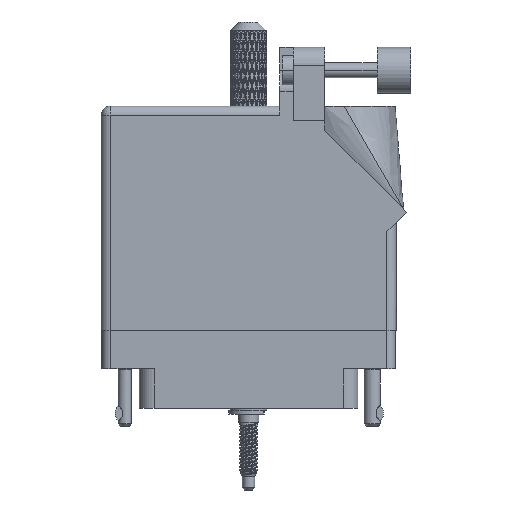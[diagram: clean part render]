
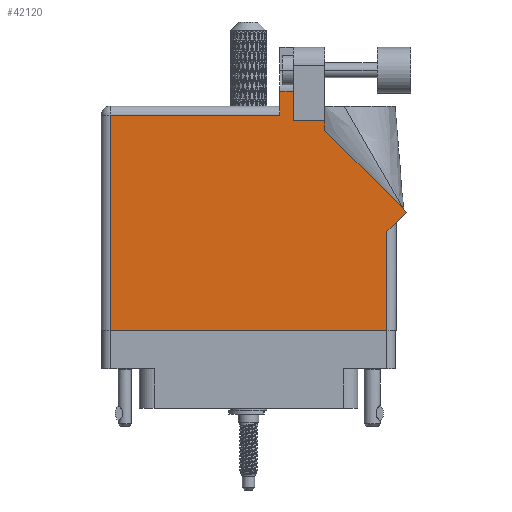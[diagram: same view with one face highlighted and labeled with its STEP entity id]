
A CAD part, front view. The second image highlights one B-rep face of the part: STEP entity #42120.
In plain terms, the highlighted face is planar.
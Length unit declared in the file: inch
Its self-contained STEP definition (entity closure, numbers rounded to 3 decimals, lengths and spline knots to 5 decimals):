
#35 = LINE ( 'NONE', #107461, #18611 ) ;
#295 = VECTOR ( 'NONE', #54217, 39.37008 ) ;
#3095 = ORIENTED_EDGE ( 'NONE', *, *, #90571, .T. ) ;
#4260 = VECTOR ( 'NONE', #101979, 39.37008 ) ;
#4283 = EDGE_CURVE ( 'NONE', #41379, #85957, #13879, .T. ) ;
#4672 = EDGE_LOOP ( 'NONE', ( #17886, #47079, #49174, #107931, #3095, #56860, #93008, #79670, #86311, #7730, #45377 ) ) ;
#5504 = EDGE_CURVE ( 'NONE', #63545, #100131, #31183, .T. ) ;
#6897 = EDGE_CURVE ( 'NONE', #9833, #75771, #57679, .T. ) ;
#7074 = DIRECTION ( 'NONE',  ( -0.707, 0.707, 0. ) ) ;
#7730 = ORIENTED_EDGE ( 'NONE', *, *, #89425, .T. ) ;
#8546 = CARTESIAN_POINT ( 'NONE',  ( 1.311, 1.6315, 0. ) ) ;
#9789 = CARTESIAN_POINT ( 'NONE',  ( 1.311, 1.43, 0. ) ) ;
#9833 = VERTEX_POINT ( 'NONE', #64422 ) ;
#13066 = CARTESIAN_POINT ( 'NONE',  ( 2.08071, 0.80771, 0. ) ) ;
#13879 = LINE ( 'NONE', #101035, #41938 ) ;
#14260 = FACE_OUTER_BOUND ( 'NONE', #4672, .T. ) ;
#17886 = ORIENTED_EDGE ( 'NONE', *, *, #5504, .T. ) ;
#18052 = DIRECTION ( 'NONE',  ( 0., 1., 0. ) ) ;
#18611 = VECTOR ( 'NONE', #90372, 39.37008 ) ;
#20107 = DIRECTION ( 'NONE',  ( 0., 0., -1. ) ) ;
#24949 = DIRECTION ( 'NONE',  ( -1., 0., 0. ) ) ;
#25776 = VECTOR ( 'NONE', #74172, 39.37008 ) ;
#29349 = CARTESIAN_POINT ( 'NONE',  ( 1.948, 0., 0. ) ) ;
#31183 = LINE ( 'NONE', #9789, #91169 ) ;
#32464 = VECTOR ( 'NONE', #33419, 39.37008 ) ;
#33419 = DIRECTION ( 'NONE',  ( -1., 0., 0. ) ) ;
#33654 = EDGE_CURVE ( 'NONE', #85957, #91461, #76544, .T. ) ;
#33769 = CARTESIAN_POINT ( 'NONE',  ( 0., 1.468, 0. ) ) ;
#35671 = EDGE_CURVE ( 'NONE', #63748, #59970, #40245, .T. ) ;
#40245 = LINE ( 'NONE', #63122, #295 ) ;
#41379 = VERTEX_POINT ( 'NONE', #47139 ) ;
#41938 = VECTOR ( 'NONE', #84261, 39.37008 ) ;
#42120 = ADVANCED_FACE ( 'NONE', ( #14260 ), #53612, .F. ) ;
#44382 = CARTESIAN_POINT ( 'NONE',  ( 1.217, 1.468, 0. ) ) ;
#45377 = ORIENTED_EDGE ( 'NONE', *, *, #84362, .T. ) ;
#45420 = CARTESIAN_POINT ( 'NONE',  ( 1.311, 1.43, 0. ) ) ;
#47079 = ORIENTED_EDGE ( 'NONE', *, *, #77019, .T. ) ;
#47139 = CARTESIAN_POINT ( 'NONE',  ( 1.217, 1.6315, 0. ) ) ;
#48373 = DIRECTION ( 'NONE',  ( -1., 0., 0. ) ) ;
#48534 = CARTESIAN_POINT ( 'NONE',  ( 0., 0., 0. ) ) ;
#49151 = CARTESIAN_POINT ( 'NONE',  ( 1.524, 1.36442, 0. ) ) ;
#49174 = ORIENTED_EDGE ( 'NONE', *, *, #4283, .T. ) ;
#53612 = PLANE ( 'NONE',  #97197 ) ;
#54217 = DIRECTION ( 'NONE',  ( 0.707, 0.707, 0. ) ) ;
#56860 = ORIENTED_EDGE ( 'NONE', *, *, #6897, .T. ) ;
#57381 = CARTESIAN_POINT ( 'NONE',  ( 2.08071, 0.80771, 0. ) ) ;
#57679 = LINE ( 'NONE', #48534, #98996 ) ;
#59598 = EDGE_CURVE ( 'NONE', #75771, #63748, #35, .T. ) ;
#59970 = VERTEX_POINT ( 'NONE', #13066 ) ;
#61467 = DIRECTION ( 'NONE',  ( -1., 0., 0. ) ) ;
#63122 = CARTESIAN_POINT ( 'NONE',  ( 2.01, 0.737, 0. ) ) ;
#63545 = VERTEX_POINT ( 'NONE', #45420 ) ;
#63748 = VERTEX_POINT ( 'NONE', #93444 ) ;
#64422 = CARTESIAN_POINT ( 'NONE',  ( 0.062, 0., 0. ) ) ;
#66461 = LINE ( 'NONE', #57381, #101136 ) ;
#68892 = CARTESIAN_POINT ( 'NONE',  ( 1.524, 1.43, 0. ) ) ;
#69588 = LINE ( 'NONE', #110540, #4260 ) ;
#71134 = CARTESIAN_POINT ( 'NONE',  ( 0., 1.53, 0. ) ) ;
#72449 = LINE ( 'NONE', #74529, #97967 ) ;
#72741 = VECTOR ( 'NONE', #24949, 39.37008 ) ;
#74172 = DIRECTION ( 'NONE',  ( 0., 1., 0. ) ) ;
#74529 = CARTESIAN_POINT ( 'NONE',  ( 1.64177, 1.6315, 0. ) ) ;
#75771 = VERTEX_POINT ( 'NONE', #29349 ) ;
#76544 = LINE ( 'NONE', #33769, #32464 ) ;
#77019 = EDGE_CURVE ( 'NONE', #100131, #41379, #72449, .T. ) ;
#79134 = LINE ( 'NONE', #49151, #25776 ) ;
#79670 = ORIENTED_EDGE ( 'NONE', *, *, #35671, .T. ) ;
#82165 = CARTESIAN_POINT ( 'NONE',  ( 0.062, 1.468, 0. ) ) ;
#83227 = DIRECTION ( 'NONE',  ( 1., 0., 0. ) ) ;
#84261 = DIRECTION ( 'NONE',  ( 0., -1., 0. ) ) ;
#84362 = EDGE_CURVE ( 'NONE', #95647, #63545, #95406, .T. ) ;
#85957 = VERTEX_POINT ( 'NONE', #44382 ) ;
#86311 = ORIENTED_EDGE ( 'NONE', *, *, #108800, .T. ) ;
#89425 = EDGE_CURVE ( 'NONE', #93301, #95647, #79134, .T. ) ;
#90372 = DIRECTION ( 'NONE',  ( 0., 1., 0. ) ) ;
#90571 = EDGE_CURVE ( 'NONE', #91461, #9833, #69588, .T. ) ;
#91169 = VECTOR ( 'NONE', #18052, 39.37008 ) ;
#91461 = VERTEX_POINT ( 'NONE', #82165 ) ;
#93008 = ORIENTED_EDGE ( 'NONE', *, *, #59598, .T. ) ;
#93301 = VERTEX_POINT ( 'NONE', #105238 ) ;
#93444 = CARTESIAN_POINT ( 'NONE',  ( 1.948, 0.675, 0. ) ) ;
#95406 = LINE ( 'NONE', #68892, #72741 ) ;
#95647 = VERTEX_POINT ( 'NONE', #107569 ) ;
#97197 = AXIS2_PLACEMENT_3D ( 'NONE', #71134, #20107, #61467 ) ;
#97967 = VECTOR ( 'NONE', #48373, 39.37008 ) ;
#98996 = VECTOR ( 'NONE', #83227, 39.37008 ) ;
#100131 = VERTEX_POINT ( 'NONE', #8546 ) ;
#101035 = CARTESIAN_POINT ( 'NONE',  ( 1.217, 1.53, 0. ) ) ;
#101136 = VECTOR ( 'NONE', #7074, 39.37008 ) ;
#101979 = DIRECTION ( 'NONE',  ( 0., -1., 0. ) ) ;
#105238 = CARTESIAN_POINT ( 'NONE',  ( 1.524, 1.36442, 0. ) ) ;
#107461 = CARTESIAN_POINT ( 'NONE',  ( 1.948, 0.737, 0. ) ) ;
#107569 = CARTESIAN_POINT ( 'NONE',  ( 1.524, 1.43, 0. ) ) ;
#107931 = ORIENTED_EDGE ( 'NONE', *, *, #33654, .T. ) ;
#108800 = EDGE_CURVE ( 'NONE', #59970, #93301, #66461, .T. ) ;
#110540 = CARTESIAN_POINT ( 'NONE',  ( 0.062, 0., 0. ) ) ;
